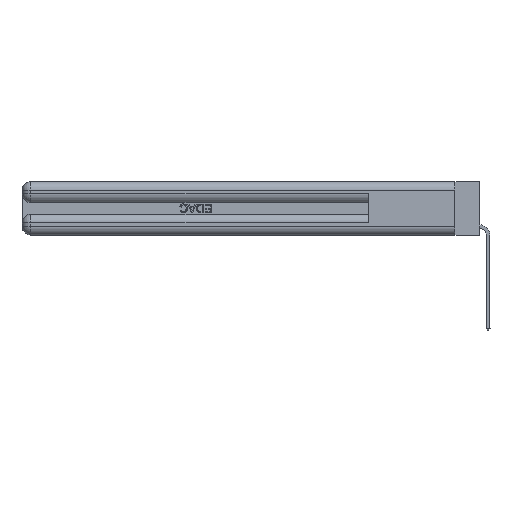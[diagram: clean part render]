
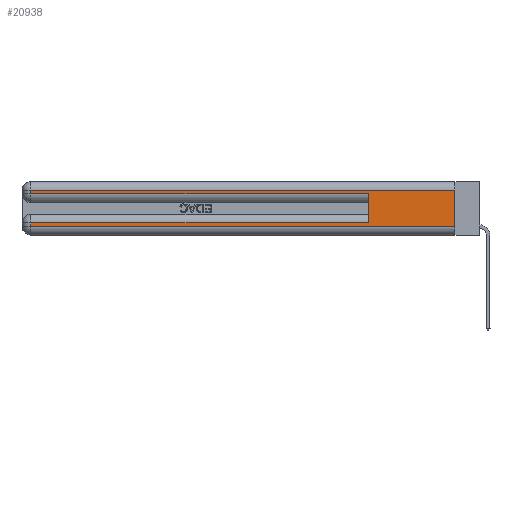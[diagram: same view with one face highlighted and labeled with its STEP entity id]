
A CAD part, left-side view. The second image highlights one B-rep face of the part: STEP entity #20938.
In plain terms, the highlighted planar face has unit normal (-1, 0, 0).
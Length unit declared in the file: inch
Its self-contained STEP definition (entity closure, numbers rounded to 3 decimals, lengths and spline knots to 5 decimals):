
#322 = EDGE_LOOP ( 'NONE', ( #10765, #14426, #11496, #4805, #29404, #10601, #8942, #24296 ) ) ;
#1440 = CARTESIAN_POINT ( 'NONE',  ( 0., 0., 0.06 ) ) ;
#2281 = DIRECTION ( 'NONE',  ( 0., 0., -1. ) ) ;
#2619 = DIRECTION ( 'NONE',  ( 0., 0., -1. ) ) ;
#3914 = VECTOR ( 'NONE', #25598, 39.37008 ) ;
#4420 = VECTOR ( 'NONE', #16689, 39.37008 ) ;
#4780 = VECTOR ( 'NONE', #2619, 39.37008 ) ;
#4805 = ORIENTED_EDGE ( 'NONE', *, *, #12171, .T. ) ;
#5687 = VECTOR ( 'NONE', #11609, 39.37008 ) ;
#6374 = PLANE ( 'NONE',  #7032 ) ;
#7032 = AXIS2_PLACEMENT_3D ( 'NONE', #13188, #22358, #8725 ) ;
#7872 = CARTESIAN_POINT ( 'NONE',  ( 0., 0., 0.31 ) ) ;
#8725 = DIRECTION ( 'NONE',  ( 0., 0., -1. ) ) ;
#8942 = ORIENTED_EDGE ( 'NONE', *, *, #15543, .T. ) ;
#9176 = VECTOR ( 'NONE', #19704, 39.37008 ) ;
#9589 = CARTESIAN_POINT ( 'NONE',  ( 0., 2.94, 0.06 ) ) ;
#10601 = ORIENTED_EDGE ( 'NONE', *, *, #14929, .T. ) ;
#10714 = EDGE_CURVE ( 'NONE', #24043, #23615, #17935, .T. ) ;
#10765 = ORIENTED_EDGE ( 'NONE', *, *, #10714, .F. ) ;
#11146 = LINE ( 'NONE', #24842, #27824 ) ;
#11496 = ORIENTED_EDGE ( 'NONE', *, *, #11936, .T. ) ;
#11609 = DIRECTION ( 'NONE',  ( 0., 0., 1. ) ) ;
#11657 = FACE_OUTER_BOUND ( 'NONE', #322, .T. ) ;
#11936 = EDGE_CURVE ( 'NONE', #19868, #17796, #11146, .T. ) ;
#12126 = VERTEX_POINT ( 'NONE', #9589 ) ;
#12171 = EDGE_CURVE ( 'NONE', #17796, #22288, #16818, .T. ) ;
#12506 = LINE ( 'NONE', #18485, #5687 ) ;
#12792 = EDGE_CURVE ( 'NONE', #12793, #22288, #12506, .T. ) ;
#12793 = VERTEX_POINT ( 'NONE', #20793 ) ;
#13007 = CARTESIAN_POINT ( 'NONE',  ( 0., 0., 0.085 ) ) ;
#13188 = CARTESIAN_POINT ( 'NONE',  ( 0., 0., 0.37 ) ) ;
#14095 = CARTESIAN_POINT ( 'NONE',  ( 0., 2.94, 0.37 ) ) ;
#14426 = ORIENTED_EDGE ( 'NONE', *, *, #21055, .T. ) ;
#14929 = EDGE_CURVE ( 'NONE', #12793, #28802, #26592, .T. ) ;
#15543 = EDGE_CURVE ( 'NONE', #28802, #12126, #16961, .T. ) ;
#15596 = VECTOR ( 'NONE', #23804, 39.37008 ) ;
#15901 = LINE ( 'NONE', #19095, #4420 ) ;
#16689 = DIRECTION ( 'NONE',  ( 0., -1., 0. ) ) ;
#16818 = LINE ( 'NONE', #21061, #3914 ) ;
#16961 = LINE ( 'NONE', #14095, #4780 ) ;
#17796 = VERTEX_POINT ( 'NONE', #18343 ) ;
#17935 = LINE ( 'NONE', #27343, #29255 ) ;
#18343 = CARTESIAN_POINT ( 'NONE',  ( 0., 2.94, 0.285 ) ) ;
#18485 = CARTESIAN_POINT ( 'NONE',  ( 0., 0.6, 0.145 ) ) ;
#19095 = CARTESIAN_POINT ( 'NONE',  ( 0., 0., 0.06 ) ) ;
#19559 = CARTESIAN_POINT ( 'NONE',  ( 0., 0., 0.31 ) ) ;
#19704 = DIRECTION ( 'NONE',  ( 0., 1., 0. ) ) ;
#19868 = VERTEX_POINT ( 'NONE', #25077 ) ;
#20793 = CARTESIAN_POINT ( 'NONE',  ( 0., 0.6, 0.085 ) ) ;
#20938 = ADVANCED_FACE ( 'NONE', ( #11657 ), #6374, .F. ) ;
#21055 = EDGE_CURVE ( 'NONE', #24043, #19868, #26940, .T. ) ;
#21060 = CARTESIAN_POINT ( 'NONE',  ( 0., 0.6, 0.285 ) ) ;
#21061 = CARTESIAN_POINT ( 'NONE',  ( 0., 0., 0.285 ) ) ;
#21697 = EDGE_CURVE ( 'NONE', #12126, #23615, #15901, .T. ) ;
#22288 = VERTEX_POINT ( 'NONE', #21060 ) ;
#22358 = DIRECTION ( 'NONE',  ( 1., 0., 0. ) ) ;
#23615 = VERTEX_POINT ( 'NONE', #1440 ) ;
#23804 = DIRECTION ( 'NONE',  ( 0., 1., 0. ) ) ;
#24043 = VERTEX_POINT ( 'NONE', #19559 ) ;
#24296 = ORIENTED_EDGE ( 'NONE', *, *, #21697, .T. ) ;
#24842 = CARTESIAN_POINT ( 'NONE',  ( 0., 2.94, 0.37 ) ) ;
#25077 = CARTESIAN_POINT ( 'NONE',  ( 0., 2.94, 0.31 ) ) ;
#25598 = DIRECTION ( 'NONE',  ( 0., -1., 0. ) ) ;
#25847 = CARTESIAN_POINT ( 'NONE',  ( 0., 2.94, 0.085 ) ) ;
#26592 = LINE ( 'NONE', #13007, #9176 ) ;
#26940 = LINE ( 'NONE', #7872, #15596 ) ;
#27093 = DIRECTION ( 'NONE',  ( 0., 0., -1. ) ) ;
#27343 = CARTESIAN_POINT ( 'NONE',  ( 0., 0., 0.37 ) ) ;
#27824 = VECTOR ( 'NONE', #27093, 39.37008 ) ;
#28802 = VERTEX_POINT ( 'NONE', #25847 ) ;
#29255 = VECTOR ( 'NONE', #2281, 39.37008 ) ;
#29404 = ORIENTED_EDGE ( 'NONE', *, *, #12792, .F. ) ;
